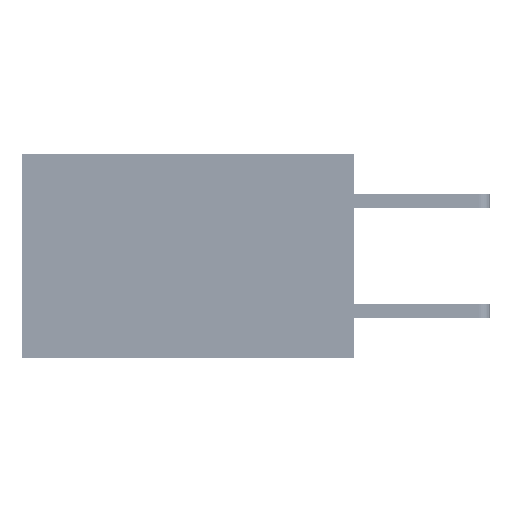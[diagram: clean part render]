
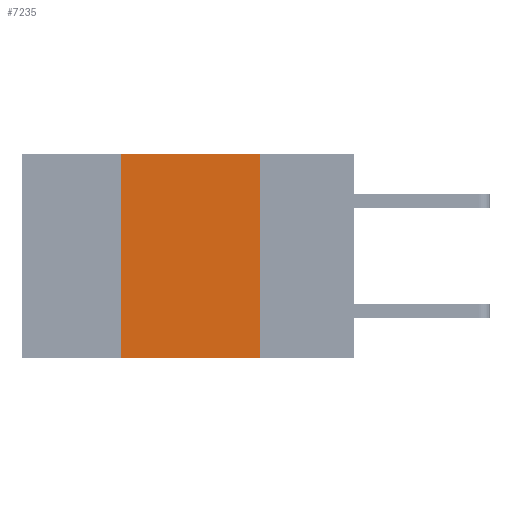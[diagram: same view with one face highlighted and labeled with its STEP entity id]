
A CAD part, left-side view. The second image highlights one B-rep face of the part: STEP entity #7235.
In plain terms, the highlighted planar face has unit normal (-1, 0, 0).
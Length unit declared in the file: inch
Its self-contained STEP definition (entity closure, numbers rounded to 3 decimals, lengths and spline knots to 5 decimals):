
#280 = VERTEX_POINT ( 'NONE', #47580 ) ;
#3114 = DIRECTION ( 'NONE',  ( 0., -1., 0. ) ) ;
#3618 = CARTESIAN_POINT ( 'NONE',  ( 0., 0.6, 0. ) ) ;
#4344 = ORIENTED_EDGE ( 'NONE', *, *, #14725, .F. ) ;
#7235 = ADVANCED_FACE ( 'NONE', ( #15779 ), #16034, .F. ) ;
#9780 = CARTESIAN_POINT ( 'NONE',  ( 0., 0.42, 0. ) ) ;
#9960 = CARTESIAN_POINT ( 'NONE',  ( 0., 0.17, 0. ) ) ;
#10378 = ORIENTED_EDGE ( 'NONE', *, *, #36766, .T. ) ;
#11145 = CARTESIAN_POINT ( 'NONE',  ( 0., 0.17, 0. ) ) ;
#14725 = EDGE_CURVE ( 'NONE', #37546, #280, #29650, .T. ) ;
#15779 = FACE_OUTER_BOUND ( 'NONE', #34957, .T. ) ;
#16034 = PLANE ( 'NONE',  #50076 ) ;
#16548 = DIRECTION ( 'NONE',  ( 1., 0., 0. ) ) ;
#19335 = EDGE_CURVE ( 'NONE', #48182, #29691, #37915, .T. ) ;
#19668 = ORIENTED_EDGE ( 'NONE', *, *, #34161, .F. ) ;
#22049 = DIRECTION ( 'NONE',  ( 0., 0., 1. ) ) ;
#23225 = LINE ( 'NONE', #3618, #44388 ) ;
#24133 = CARTESIAN_POINT ( 'NONE',  ( 0., 0.6, 0. ) ) ;
#25372 = DIRECTION ( 'NONE',  ( 0., 0., -1. ) ) ;
#29650 = LINE ( 'NONE', #9780, #35800 ) ;
#29691 = VERTEX_POINT ( 'NONE', #50008 ) ;
#29711 = CARTESIAN_POINT ( 'NONE',  ( 0., 0.42, -0.37 ) ) ;
#30653 = LINE ( 'NONE', #34824, #46159 ) ;
#34161 = EDGE_CURVE ( 'NONE', #280, #48182, #23225, .T. ) ;
#34824 = CARTESIAN_POINT ( 'NONE',  ( 0., 0.6, -0.37 ) ) ;
#34957 = EDGE_LOOP ( 'NONE', ( #46758, #19668, #4344, #10378 ) ) ;
#35800 = VECTOR ( 'NONE', #22049, 39.37008 ) ;
#36766 = EDGE_CURVE ( 'NONE', #37546, #29691, #30653, .T. ) ;
#37546 = VERTEX_POINT ( 'NONE', #29711 ) ;
#37915 = LINE ( 'NONE', #9960, #50489 ) ;
#38231 = DIRECTION ( 'NONE',  ( 0., -1., 0. ) ) ;
#44388 = VECTOR ( 'NONE', #3114, 39.37008 ) ;
#46159 = VECTOR ( 'NONE', #38231, 39.37008 ) ;
#46758 = ORIENTED_EDGE ( 'NONE', *, *, #19335, .F. ) ;
#47580 = CARTESIAN_POINT ( 'NONE',  ( 0., 0.42, 0. ) ) ;
#47691 = DIRECTION ( 'NONE',  ( 0., 0., -1. ) ) ;
#48182 = VERTEX_POINT ( 'NONE', #11145 ) ;
#50008 = CARTESIAN_POINT ( 'NONE',  ( 0., 0.17, -0.37 ) ) ;
#50076 = AXIS2_PLACEMENT_3D ( 'NONE', #24133, #16548, #47691 ) ;
#50489 = VECTOR ( 'NONE', #25372, 39.37008 ) ;
